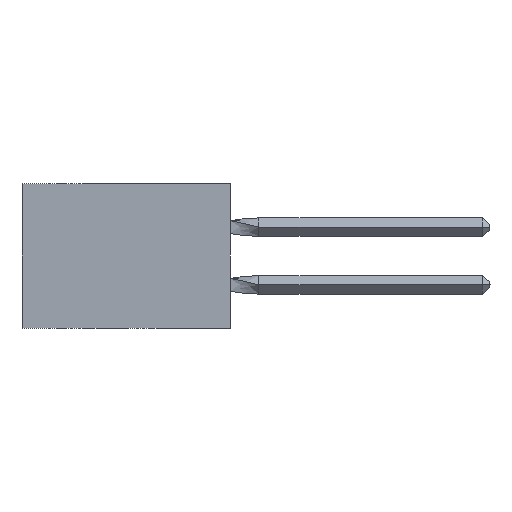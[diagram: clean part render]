
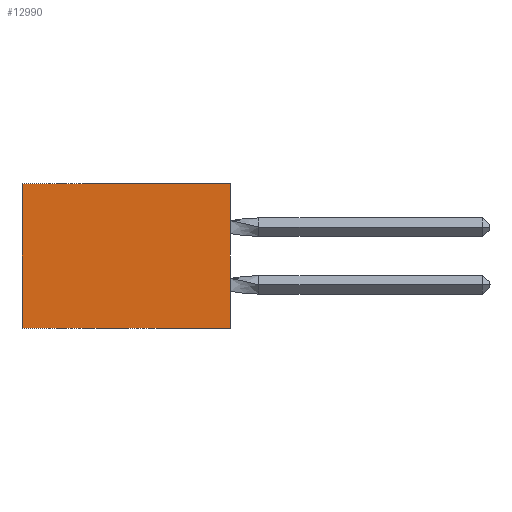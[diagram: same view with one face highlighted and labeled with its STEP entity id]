
A CAD part, left-side view. The second image highlights one B-rep face of the part: STEP entity #12990.
In plain terms, the highlighted planar face has unit normal (-1, 0, 0).
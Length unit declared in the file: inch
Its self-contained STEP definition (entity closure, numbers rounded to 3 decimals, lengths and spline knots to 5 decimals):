
#194 = CARTESIAN_POINT ( 'NONE',  ( 0.305, 0., -0.5 ) ) ;
#309 = CARTESIAN_POINT ( 'NONE',  ( 0.305, 0., 0. ) ) ;
#580 = FACE_OUTER_BOUND ( 'NONE', #13721, .T. ) ;
#753 = DIRECTION ( 'NONE',  ( 0., 1., 0. ) ) ;
#1325 = AXIS2_PLACEMENT_3D ( 'NONE', #8197, #14028, #11744 ) ;
#2187 = VERTEX_POINT ( 'NONE', #11425 ) ;
#2588 = LINE ( 'NONE', #309, #14206 ) ;
#2760 = VERTEX_POINT ( 'NONE', #194 ) ;
#3628 = VECTOR ( 'NONE', #12158, 39.37008 ) ;
#3690 = CARTESIAN_POINT ( 'NONE',  ( 0.305, 0., -0.5 ) ) ;
#3726 = DIRECTION ( 'NONE',  ( 0., 1., 0. ) ) ;
#4504 = EDGE_CURVE ( 'NONE', #2187, #8455, #12618, .T. ) ;
#4972 = ORIENTED_EDGE ( 'NONE', *, *, #7215, .T. ) ;
#5014 = CARTESIAN_POINT ( 'NONE',  ( 0.305, 0., 0. ) ) ;
#5194 = ORIENTED_EDGE ( 'NONE', *, *, #7494, .F. ) ;
#6503 = ORIENTED_EDGE ( 'NONE', *, *, #4504, .T. ) ;
#6571 = LINE ( 'NONE', #8605, #9941 ) ;
#7215 = EDGE_CURVE ( 'NONE', #14434, #2187, #2588, .T. ) ;
#7247 = LINE ( 'NONE', #3690, #13913 ) ;
#7494 = EDGE_CURVE ( 'NONE', #2760, #8455, #6571, .T. ) ;
#8197 = CARTESIAN_POINT ( 'NONE',  ( 0.305, 0., -0.5 ) ) ;
#8455 = VERTEX_POINT ( 'NONE', #9436 ) ;
#8605 = CARTESIAN_POINT ( 'NONE',  ( 0.305, 0., -0.5 ) ) ;
#8996 = EDGE_CURVE ( 'NONE', #14434, #2760, #7247, .T. ) ;
#9436 = CARTESIAN_POINT ( 'NONE',  ( 0.305, 0.72, -0.5 ) ) ;
#9490 = PLANE ( 'NONE',  #1325 ) ;
#9941 = VECTOR ( 'NONE', #753, 39.37008 ) ;
#11425 = CARTESIAN_POINT ( 'NONE',  ( 0.305, 0.72, 0. ) ) ;
#11744 = DIRECTION ( 'NONE',  ( 0., 0., -1. ) ) ;
#12158 = DIRECTION ( 'NONE',  ( 0., 0., -1. ) ) ;
#12618 = LINE ( 'NONE', #13272, #3628 ) ;
#12800 = DIRECTION ( 'NONE',  ( 0., 0., -1. ) ) ;
#12990 = ADVANCED_FACE ( 'NONE', ( #580 ), #9490, .F. ) ;
#13272 = CARTESIAN_POINT ( 'NONE',  ( 0.305, 0.72, -0.5 ) ) ;
#13548 = ORIENTED_EDGE ( 'NONE', *, *, #8996, .F. ) ;
#13721 = EDGE_LOOP ( 'NONE', ( #6503, #5194, #13548, #4972 ) ) ;
#13913 = VECTOR ( 'NONE', #12800, 39.37008 ) ;
#14028 = DIRECTION ( 'NONE',  ( 1., 0., 0. ) ) ;
#14206 = VECTOR ( 'NONE', #3726, 39.37008 ) ;
#14434 = VERTEX_POINT ( 'NONE', #5014 ) ;
